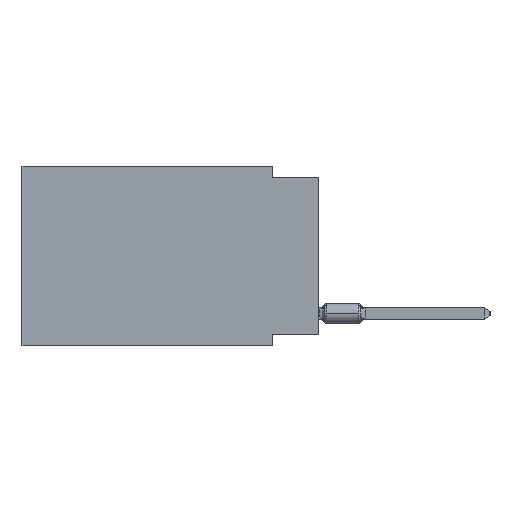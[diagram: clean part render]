
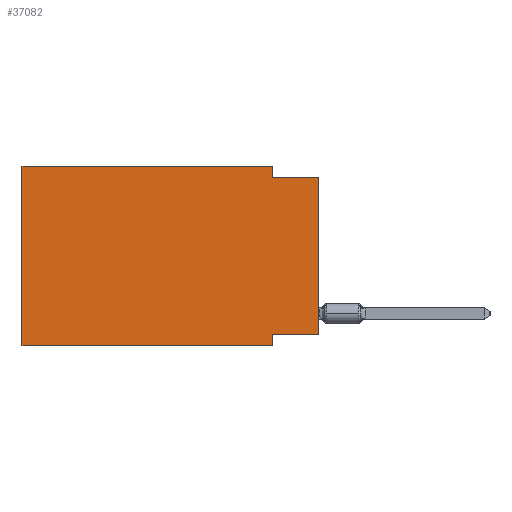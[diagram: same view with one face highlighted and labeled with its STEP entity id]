
A CAD part, left-side view. The second image highlights one B-rep face of the part: STEP entity #37082.
In plain terms, the highlighted planar face has unit normal (-1, 0, 0).
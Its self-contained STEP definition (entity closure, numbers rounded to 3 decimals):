
#424 = CARTESIAN_POINT ( 'NONE',  ( 0., 2.54, 0. ) ) ;
#815 = DIRECTION ( 'NONE',  ( 0., 1., 0. ) ) ;
#883 = CARTESIAN_POINT ( 'NONE',  ( 0., 16.383, 0. ) ) ;
#2612 = ORIENTED_EDGE ( 'NONE', *, *, #41720, .T. ) ;
#4353 = VECTOR ( 'NONE', #13989, 1000. ) ;
#5004 = CARTESIAN_POINT ( 'NONE',  ( 0., 2.54, -9.906 ) ) ;
#6667 = EDGE_CURVE ( 'NONE', #41484, #49024, #16926, .T. ) ;
#7311 = EDGE_CURVE ( 'NONE', #49024, #22896, #32629, .T. ) ;
#9076 = CARTESIAN_POINT ( 'NONE',  ( 0., 0., -9.271 ) ) ;
#10614 = LINE ( 'NONE', #22893, #16641 ) ;
#11311 = ORIENTED_EDGE ( 'NONE', *, *, #48423, .T. ) ;
#11364 = CARTESIAN_POINT ( 'NONE',  ( 0., 2.54, -9.906 ) ) ;
#12034 = DIRECTION ( 'NONE',  ( 0., 0., 1. ) ) ;
#13276 = ORIENTED_EDGE ( 'NONE', *, *, #44800, .F. ) ;
#13423 = AXIS2_PLACEMENT_3D ( 'NONE', #883, #17523, #21343 ) ;
#13989 = DIRECTION ( 'NONE',  ( 0., 0., -1. ) ) ;
#14555 = VERTEX_POINT ( 'NONE', #35834 ) ;
#14977 = DIRECTION ( 'NONE',  ( 0., -1., 0. ) ) ;
#15106 = ORIENTED_EDGE ( 'NONE', *, *, #31521, .F. ) ;
#15753 = EDGE_CURVE ( 'NONE', #18425, #48249, #49525, .T. ) ;
#15880 = LINE ( 'NONE', #16935, #28951 ) ;
#16581 = CARTESIAN_POINT ( 'NONE',  ( 0., 2.54, -9.271 ) ) ;
#16641 = VECTOR ( 'NONE', #14977, 1000. ) ;
#16838 = CARTESIAN_POINT ( 'NONE',  ( 0., 16.383, 0. ) ) ;
#16926 = LINE ( 'NONE', #29980, #52471 ) ;
#16935 = CARTESIAN_POINT ( 'NONE',  ( 0., 0., 0. ) ) ;
#17358 = ORIENTED_EDGE ( 'NONE', *, *, #15753, .F. ) ;
#17523 = DIRECTION ( 'NONE',  ( 1., 0., 0. ) ) ;
#17885 = EDGE_CURVE ( 'NONE', #48249, #39724, #10614, .T. ) ;
#18425 = VERTEX_POINT ( 'NONE', #51687 ) ;
#20315 = LINE ( 'NONE', #26273, #4353 ) ;
#21096 = ORIENTED_EDGE ( 'NONE', *, *, #7311, .F. ) ;
#21343 = DIRECTION ( 'NONE',  ( 0., 0., -1. ) ) ;
#22219 = CARTESIAN_POINT ( 'NONE',  ( 0., 16.383, 0. ) ) ;
#22893 = CARTESIAN_POINT ( 'NONE',  ( 0., 16.383, 0. ) ) ;
#22896 = VERTEX_POINT ( 'NONE', #5004 ) ;
#24756 = VERTEX_POINT ( 'NONE', #39648 ) ;
#26273 = CARTESIAN_POINT ( 'NONE',  ( 0., 2.54, 0. ) ) ;
#27654 = DIRECTION ( 'NONE',  ( 0., -1., 0. ) ) ;
#28169 = ORIENTED_EDGE ( 'NONE', *, *, #6667, .F. ) ;
#28641 = VECTOR ( 'NONE', #50317, 1000. ) ;
#28951 = VECTOR ( 'NONE', #12034, 1000. ) ;
#29239 = FACE_OUTER_BOUND ( 'NONE', #41015, .T. ) ;
#29761 = VECTOR ( 'NONE', #27654, 1000. ) ;
#29980 = CARTESIAN_POINT ( 'NONE',  ( 0., 0., -9.271 ) ) ;
#30097 = LINE ( 'NONE', #41829, #45845 ) ;
#31521 = EDGE_CURVE ( 'NONE', #39724, #14555, #20315, .T. ) ;
#32629 = LINE ( 'NONE', #11364, #52512 ) ;
#35834 = CARTESIAN_POINT ( 'NONE',  ( 0., 2.54, -0.635 ) ) ;
#37082 = ADVANCED_FACE ( 'NONE', ( #29239 ), #45876, .F. ) ;
#38857 = ORIENTED_EDGE ( 'NONE', *, *, #17885, .F. ) ;
#39648 = CARTESIAN_POINT ( 'NONE',  ( 0., 0., -0.635 ) ) ;
#39724 = VERTEX_POINT ( 'NONE', #424 ) ;
#40188 = LINE ( 'NONE', #47550, #29761 ) ;
#41015 = EDGE_LOOP ( 'NONE', ( #2612, #13276, #15106, #38857, #17358, #11311, #21096, #28169 ) ) ;
#41484 = VERTEX_POINT ( 'NONE', #9076 ) ;
#41720 = EDGE_CURVE ( 'NONE', #41484, #24756, #15880, .T. ) ;
#41829 = CARTESIAN_POINT ( 'NONE',  ( 0., 0., -0.635 ) ) ;
#42101 = DIRECTION ( 'NONE',  ( 0., -1., 0. ) ) ;
#44800 = EDGE_CURVE ( 'NONE', #14555, #24756, #30097, .T. ) ;
#45157 = DIRECTION ( 'NONE',  ( 0., 0., -1. ) ) ;
#45845 = VECTOR ( 'NONE', #42101, 1000. ) ;
#45876 = PLANE ( 'NONE',  #13423 ) ;
#47550 = CARTESIAN_POINT ( 'NONE',  ( 0., 16.383, -9.906 ) ) ;
#48249 = VERTEX_POINT ( 'NONE', #22219 ) ;
#48423 = EDGE_CURVE ( 'NONE', #18425, #22896, #40188, .T. ) ;
#49024 = VERTEX_POINT ( 'NONE', #16581 ) ;
#49525 = LINE ( 'NONE', #16838, #28641 ) ;
#50317 = DIRECTION ( 'NONE',  ( 0., 0., 1. ) ) ;
#51687 = CARTESIAN_POINT ( 'NONE',  ( 0., 16.383, -9.906 ) ) ;
#52471 = VECTOR ( 'NONE', #815, 1000. ) ;
#52512 = VECTOR ( 'NONE', #45157, 1000. ) ;
